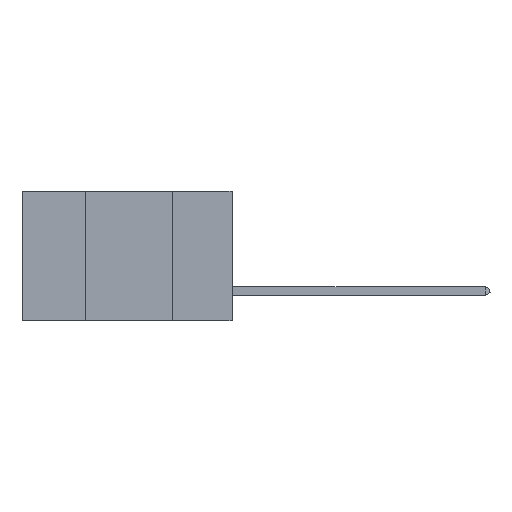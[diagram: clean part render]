
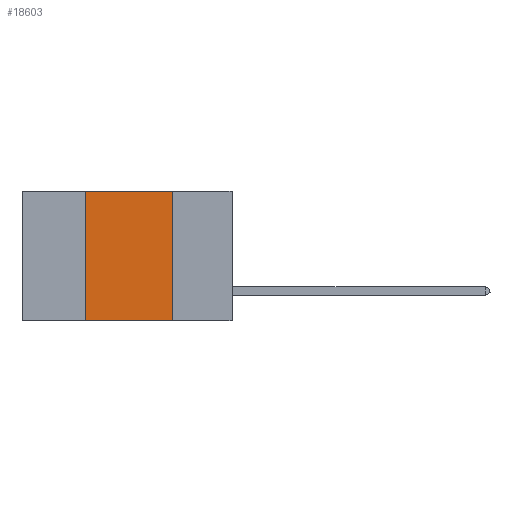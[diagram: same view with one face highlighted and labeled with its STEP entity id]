
A CAD part, left-side view. The second image highlights one B-rep face of the part: STEP entity #18603.
In plain terms, the highlighted planar face has unit normal (-1, 0, 0).
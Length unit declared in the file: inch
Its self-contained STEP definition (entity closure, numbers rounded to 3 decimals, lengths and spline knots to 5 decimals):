
#631 = CARTESIAN_POINT ( 'NONE',  ( 0., 0.6, -0.37 ) ) ;
#1965 = EDGE_LOOP ( 'NONE', ( #12924, #12933, #18350, #18511 ) ) ;
#2228 = CARTESIAN_POINT ( 'NONE',  ( 0., 0.17, -0.37 ) ) ;
#2738 = VECTOR ( 'NONE', #9705, 39.37008 ) ;
#3085 = VERTEX_POINT ( 'NONE', #20862 ) ;
#4029 = VECTOR ( 'NONE', #10196, 39.37008 ) ;
#4058 = DIRECTION ( 'NONE',  ( 0., 0., -1. ) ) ;
#4359 = DIRECTION ( 'NONE',  ( 0., -1., 0. ) ) ;
#4735 = EDGE_CURVE ( 'NONE', #3085, #6721, #8211, .T. ) ;
#5506 = EDGE_CURVE ( 'NONE', #15454, #8791, #17773, .T. ) ;
#5630 = DIRECTION ( 'NONE',  ( 0., 0., -1. ) ) ;
#6721 = VERTEX_POINT ( 'NONE', #2228 ) ;
#7099 = AXIS2_PLACEMENT_3D ( 'NONE', #10867, #12677, #5630 ) ;
#8211 = LINE ( 'NONE', #14498, #14588 ) ;
#8791 = VERTEX_POINT ( 'NONE', #12055 ) ;
#9705 = DIRECTION ( 'NONE',  ( 0., -1., 0. ) ) ;
#10196 = DIRECTION ( 'NONE',  ( 0., 0., 1. ) ) ;
#10613 = FACE_OUTER_BOUND ( 'NONE', #1965, .T. ) ;
#10867 = CARTESIAN_POINT ( 'NONE',  ( 0., 0.6, 0. ) ) ;
#12055 = CARTESIAN_POINT ( 'NONE',  ( 0., 0.42, 0. ) ) ;
#12677 = DIRECTION ( 'NONE',  ( 1., 0., 0. ) ) ;
#12924 = ORIENTED_EDGE ( 'NONE', *, *, #4735, .F. ) ;
#12933 = ORIENTED_EDGE ( 'NONE', *, *, #16065, .F. ) ;
#13360 = CARTESIAN_POINT ( 'NONE',  ( 0., 0.6, 0. ) ) ;
#14498 = CARTESIAN_POINT ( 'NONE',  ( 0., 0.17, 0. ) ) ;
#14588 = VECTOR ( 'NONE', #4058, 39.37008 ) ;
#15454 = VERTEX_POINT ( 'NONE', #20942 ) ;
#16065 = EDGE_CURVE ( 'NONE', #8791, #3085, #17869, .T. ) ;
#17773 = LINE ( 'NONE', #22472, #4029 ) ;
#17869 = LINE ( 'NONE', #13360, #2738 ) ;
#18350 = ORIENTED_EDGE ( 'NONE', *, *, #5506, .F. ) ;
#18511 = ORIENTED_EDGE ( 'NONE', *, *, #21394, .T. ) ;
#18603 = ADVANCED_FACE ( 'NONE', ( #10613 ), #21444, .F. ) ;
#20862 = CARTESIAN_POINT ( 'NONE',  ( 0., 0.17, 0. ) ) ;
#20942 = CARTESIAN_POINT ( 'NONE',  ( 0., 0.42, -0.37 ) ) ;
#21394 = EDGE_CURVE ( 'NONE', #15454, #6721, #22577, .T. ) ;
#21444 = PLANE ( 'NONE',  #7099 ) ;
#22032 = VECTOR ( 'NONE', #4359, 39.37008 ) ;
#22472 = CARTESIAN_POINT ( 'NONE',  ( 0., 0.42, 0. ) ) ;
#22577 = LINE ( 'NONE', #631, #22032 ) ;
